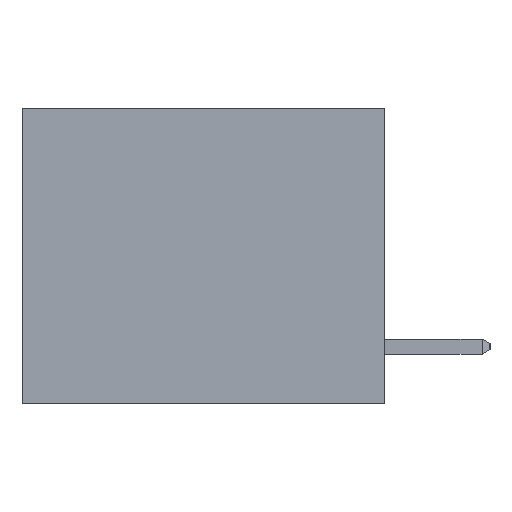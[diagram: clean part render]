
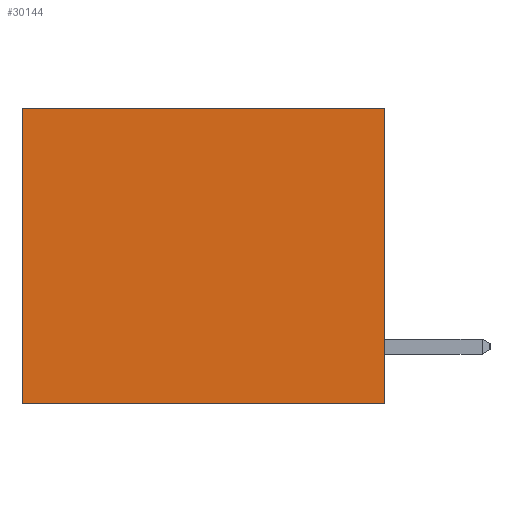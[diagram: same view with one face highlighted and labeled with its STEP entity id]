
A CAD part, left-side view. The second image highlights one B-rep face of the part: STEP entity #30144.
In plain terms, the highlighted planar face has unit normal (-1, 0, 0).
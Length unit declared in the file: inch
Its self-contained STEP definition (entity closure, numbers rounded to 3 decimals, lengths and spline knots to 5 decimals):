
#26 = CARTESIAN_POINT ( 'NONE',  ( 0.3165, 0., 0. ) ) ;
#1001 = VECTOR ( 'NONE', #26242, 39.37008 ) ;
#2171 = ORIENTED_EDGE ( 'NONE', *, *, #17028, .T. ) ;
#3403 = ORIENTED_EDGE ( 'NONE', *, *, #27308, .T. ) ;
#3511 = EDGE_LOOP ( 'NONE', ( #2171, #17241, #26287, #3403 ) ) ;
#3603 = EDGE_CURVE ( 'NONE', #28018, #10325, #23207, .T. ) ;
#5711 = VECTOR ( 'NONE', #20431, 39.37008 ) ;
#9680 = CARTESIAN_POINT ( 'NONE',  ( 0.3165, 0., 0. ) ) ;
#10325 = VERTEX_POINT ( 'NONE', #18563 ) ;
#11205 = LINE ( 'NONE', #22513, #16054 ) ;
#14003 = DIRECTION ( 'NONE',  ( 0., 0., -1. ) ) ;
#14005 = VERTEX_POINT ( 'NONE', #19357 ) ;
#15541 = CARTESIAN_POINT ( 'NONE',  ( 0.3165, 0.6, -0.49 ) ) ;
#16054 = VECTOR ( 'NONE', #19920, 39.37008 ) ;
#16430 = CARTESIAN_POINT ( 'NONE',  ( 0.3165, 0., -0.49 ) ) ;
#17028 = EDGE_CURVE ( 'NONE', #28458, #14005, #27884, .T. ) ;
#17241 = ORIENTED_EDGE ( 'NONE', *, *, #23984, .F. ) ;
#18563 = CARTESIAN_POINT ( 'NONE',  ( 0.3165, 0., -0.49 ) ) ;
#19087 = CARTESIAN_POINT ( 'NONE',  ( 0.3165, 0.6, 0. ) ) ;
#19357 = CARTESIAN_POINT ( 'NONE',  ( 0.3165, 0.6, -0.49 ) ) ;
#19516 = DIRECTION ( 'NONE',  ( 1., 0., 0. ) ) ;
#19920 = DIRECTION ( 'NONE',  ( 0., 1., 0. ) ) ;
#20431 = DIRECTION ( 'NONE',  ( 0., 0., -1. ) ) ;
#22012 = DIRECTION ( 'NONE',  ( 0., 0., -1. ) ) ;
#22105 = PLANE ( 'NONE',  #25596 ) ;
#22513 = CARTESIAN_POINT ( 'NONE',  ( 0.3165, 0., -0.49 ) ) ;
#23207 = LINE ( 'NONE', #16430, #27617 ) ;
#23984 = EDGE_CURVE ( 'NONE', #10325, #14005, #11205, .T. ) ;
#24471 = CARTESIAN_POINT ( 'NONE',  ( 0.3165, 0., -0.49 ) ) ;
#25596 = AXIS2_PLACEMENT_3D ( 'NONE', #24471, #19516, #22012 ) ;
#26242 = DIRECTION ( 'NONE',  ( 0., 1., 0. ) ) ;
#26287 = ORIENTED_EDGE ( 'NONE', *, *, #3603, .F. ) ;
#26928 = LINE ( 'NONE', #9680, #1001 ) ;
#27308 = EDGE_CURVE ( 'NONE', #28018, #28458, #26928, .T. ) ;
#27617 = VECTOR ( 'NONE', #14003, 39.37008 ) ;
#27884 = LINE ( 'NONE', #15541, #5711 ) ;
#28018 = VERTEX_POINT ( 'NONE', #26 ) ;
#28458 = VERTEX_POINT ( 'NONE', #19087 ) ;
#30144 = ADVANCED_FACE ( 'NONE', ( #30284 ), #22105, .F. ) ;
#30284 = FACE_OUTER_BOUND ( 'NONE', #3511, .T. ) ;
